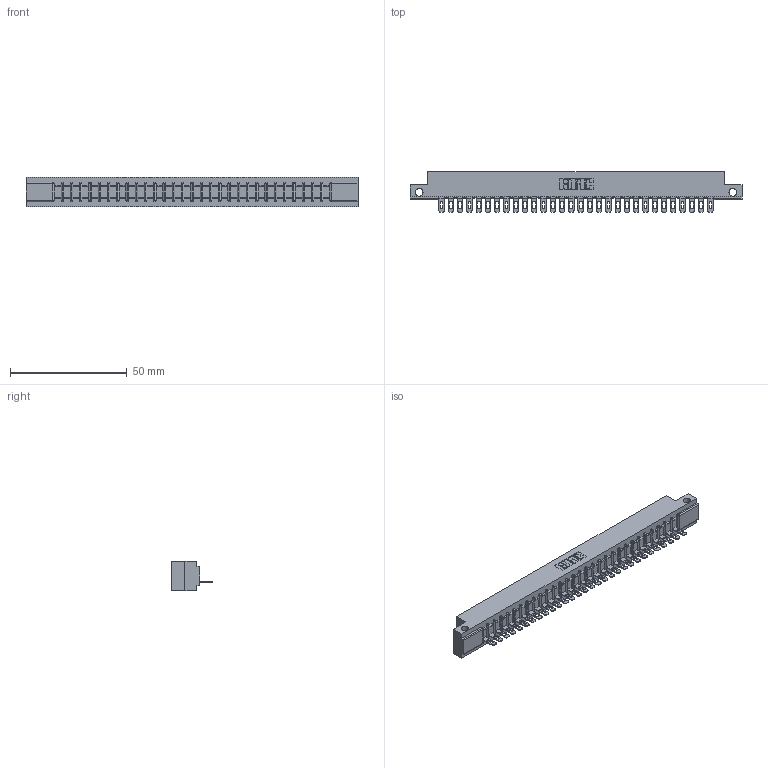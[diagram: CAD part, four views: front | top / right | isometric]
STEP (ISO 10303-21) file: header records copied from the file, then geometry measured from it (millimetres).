
FILE_DESCRIPTION (( 'STEP AP203' ), '1' );
FILE_NAME ('307-030-401-112.STEP', '2020-09-28T11:36:51', ( '' ), ( '' ), 'SwSTEP 2.0', 'SolidWorks 2020', '' );
FILE_SCHEMA (( 'CONFIG_CONTROL_DESIGN' ));
Length unit declared in the file: inch
Products named in the file (3): 307-030-401-112; 307 Part_.128 Dia Side Mounting Holes; 307-290-002_501
Assembly tree (31 placements, depth 2):
  307-030-401-112
    307 Part_.128 Dia Side Mounting Holes
    307-290-002_501  x30
Bounding box: 141.88 x 17.42 x 12.7 mm (x, y, z)
Volume: 14978 mm3; surface area: 18761.7 mm2
Topology: 31 solids, 31 shells, 2429 faces, 7463 edges, 4890 vertices
Faces by surface type: plane 1390, cylinder 977, sphere 62
Entity records: 27994 total; most frequent: CARTESIAN_POINT 4720, ORIENTED_EDGE 4710, DIRECTION 4595, EDGE_CURVE 2355, LINE 1793, VECTOR 1793, VERTEX_POINT 1526, AXIS2_PLACEMENT_3D 1401
